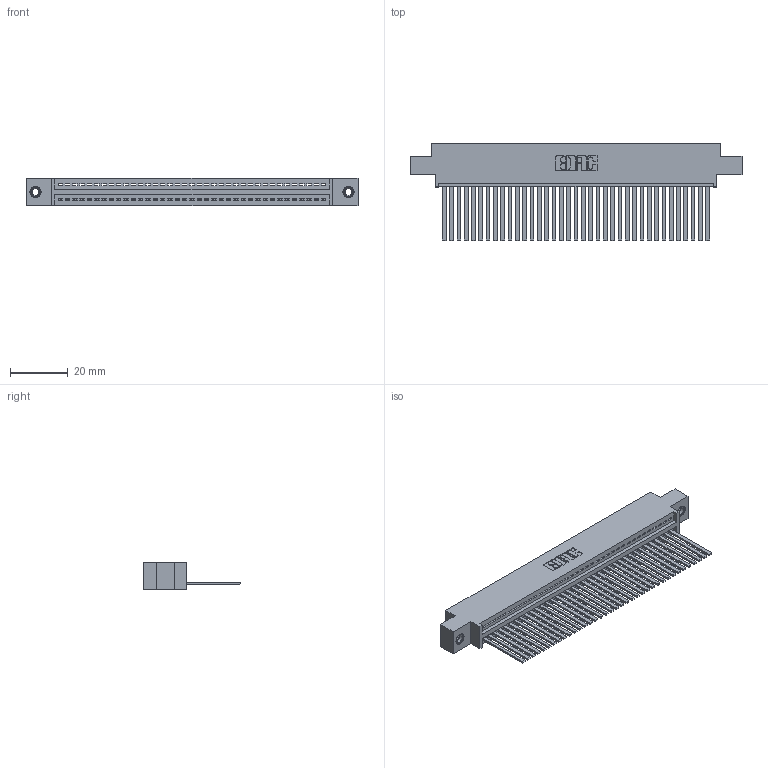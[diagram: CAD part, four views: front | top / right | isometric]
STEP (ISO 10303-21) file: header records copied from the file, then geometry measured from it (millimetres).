
FILE_DESCRIPTION (( 'STEP AP203' ), '1' );
FILE_NAME ('345-037-544-608.STEP', '2019-10-08T02:15:01', ( '' ), ( '' ), 'SwSTEP 2.0', 'SolidWorks 2016', '' );
FILE_SCHEMA (( 'CONFIG_CONTROL_DESIGN' ));
Length unit declared in the file: inch
Products named in the file (4): 345-250-001_345-250-003-102; 345-037-544-608; 345 Part_0.170 Offset - 0.156 Dia-TI; 345-292-001_345-293-144
Assembly tree (40 placements, depth 2):
  345-037-544-608
    345 Part_0.170 Offset - 0.156 Dia-TI
    345-292-001_345-293-144  x37
    345-250-001_345-250-003-102  x2
Bounding box: 115.19 x 33.96 x 9.4 mm (x, y, z)
Volume: 11208.4 mm3; surface area: 16259.1 mm2
Topology: 40 solids, 40 shells, 2114 faces, 6335 edges, 4166 vertices
Faces by surface type: plane 1448, cylinder 650, cone 12, torus 4
Entity records: 29654 total; most frequent: CARTESIAN_POINT 5118, ORIENTED_EDGE 5082, DIRECTION 4501, EDGE_CURVE 2541, VECTOR 2245, LINE 2245, VERTEX_POINT 1688, AXIS2_PLACEMENT_3D 1128
